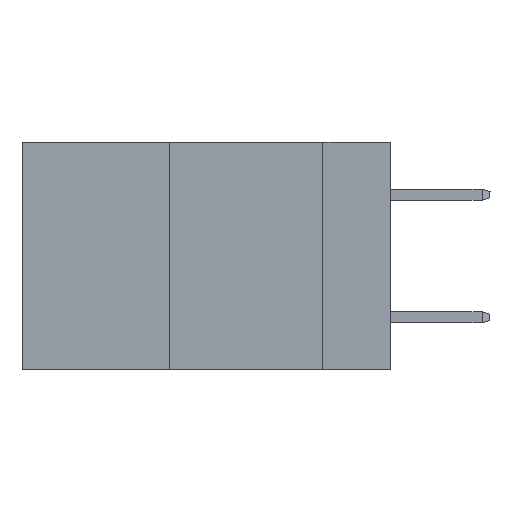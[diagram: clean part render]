
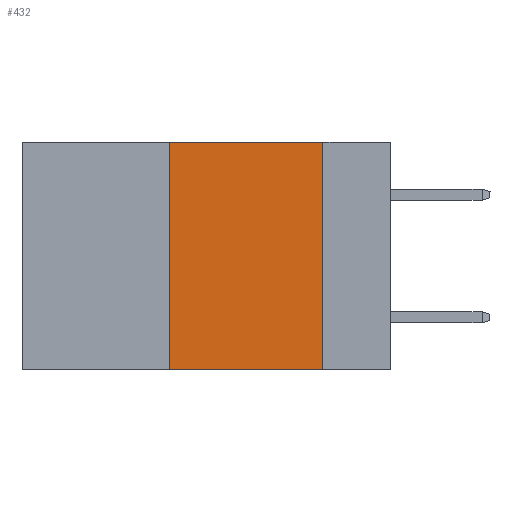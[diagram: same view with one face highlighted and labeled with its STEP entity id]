
A CAD part, left-side view. The second image highlights one B-rep face of the part: STEP entity #432.
In plain terms, the highlighted planar face has unit normal (-1, 0, 0).
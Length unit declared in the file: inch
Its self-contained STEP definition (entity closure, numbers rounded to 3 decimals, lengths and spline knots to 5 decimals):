
#25 = DIRECTION ( 'NONE',  ( 0., -1., 0. ) ) ;
#169 = VERTEX_POINT ( 'NONE', #3383 ) ;
#379 = DIRECTION ( 'NONE',  ( 0., -1., 0. ) ) ;
#432 = ADVANCED_FACE ( 'NONE', ( #5709 ), #1447, .F. ) ;
#761 = LINE ( 'NONE', #11769, #17004 ) ;
#1447 = PLANE ( 'NONE',  #3994 ) ;
#1526 = DIRECTION ( 'NONE',  ( 0., 0., -1. ) ) ;
#2012 = LINE ( 'NONE', #7576, #2847 ) ;
#2060 = ORIENTED_EDGE ( 'NONE', *, *, #14571, .F. ) ;
#2847 = VECTOR ( 'NONE', #379, 39.37008 ) ;
#3383 = CARTESIAN_POINT ( 'NONE',  ( 0., 0.36, 0. ) ) ;
#3994 = AXIS2_PLACEMENT_3D ( 'NONE', #16568, #14110, #1526 ) ;
#4062 = VECTOR ( 'NONE', #25, 39.37008 ) ;
#4244 = CARTESIAN_POINT ( 'NONE',  ( 0., 0.36, 0. ) ) ;
#5057 = CARTESIAN_POINT ( 'NONE',  ( 0., 0.11, 0. ) ) ;
#5338 = EDGE_CURVE ( 'NONE', #8986, #16973, #17060, .T. ) ;
#5709 = FACE_OUTER_BOUND ( 'NONE', #8226, .T. ) ;
#7576 = CARTESIAN_POINT ( 'NONE',  ( 0., 0.6, 0. ) ) ;
#8226 = EDGE_LOOP ( 'NONE', ( #15284, #2060, #11249, #10063 ) ) ;
#8986 = VERTEX_POINT ( 'NONE', #11233 ) ;
#9181 = EDGE_CURVE ( 'NONE', #16927, #16973, #761, .T. ) ;
#9595 = DIRECTION ( 'NONE',  ( 0., 0., 1. ) ) ;
#9692 = EDGE_CURVE ( 'NONE', #8986, #169, #12357, .T. ) ;
#10030 = VECTOR ( 'NONE', #9595, 39.37008 ) ;
#10063 = ORIENTED_EDGE ( 'NONE', *, *, #5338, .T. ) ;
#11233 = CARTESIAN_POINT ( 'NONE',  ( 0., 0.36, -0.37 ) ) ;
#11249 = ORIENTED_EDGE ( 'NONE', *, *, #9692, .F. ) ;
#11769 = CARTESIAN_POINT ( 'NONE',  ( 0., 0.11, 0. ) ) ;
#12357 = LINE ( 'NONE', #4244, #10030 ) ;
#13244 = DIRECTION ( 'NONE',  ( 0., 0., -1. ) ) ;
#14110 = DIRECTION ( 'NONE',  ( 1., 0., 0. ) ) ;
#14571 = EDGE_CURVE ( 'NONE', #169, #16927, #2012, .T. ) ;
#15284 = ORIENTED_EDGE ( 'NONE', *, *, #9181, .F. ) ;
#16348 = CARTESIAN_POINT ( 'NONE',  ( 0., 0.11, -0.37 ) ) ;
#16568 = CARTESIAN_POINT ( 'NONE',  ( 0., 0.6, 0. ) ) ;
#16875 = CARTESIAN_POINT ( 'NONE',  ( 0., 0.6, -0.37 ) ) ;
#16927 = VERTEX_POINT ( 'NONE', #5057 ) ;
#16973 = VERTEX_POINT ( 'NONE', #16348 ) ;
#17004 = VECTOR ( 'NONE', #13244, 39.37008 ) ;
#17060 = LINE ( 'NONE', #16875, #4062 ) ;
